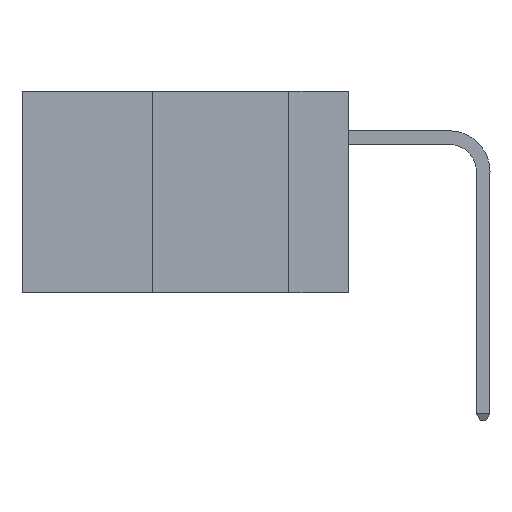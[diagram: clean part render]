
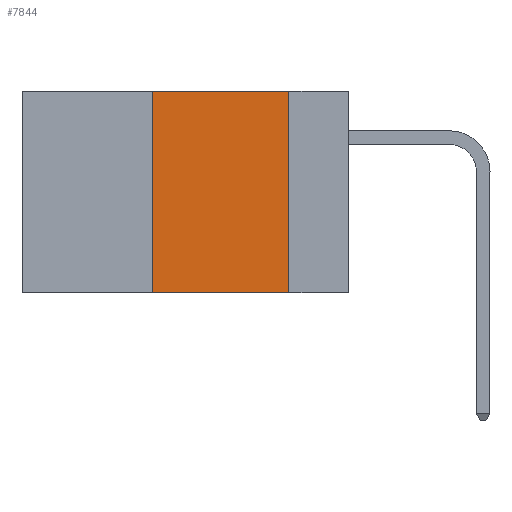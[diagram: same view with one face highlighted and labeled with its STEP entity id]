
A CAD part, left-side view. The second image highlights one B-rep face of the part: STEP entity #7844.
In plain terms, the highlighted planar face has unit normal (-1, 0, 0).
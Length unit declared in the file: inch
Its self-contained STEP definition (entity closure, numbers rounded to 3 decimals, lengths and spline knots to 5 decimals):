
#336 = ORIENTED_EDGE ( 'NONE', *, *, #8091, .F. ) ;
#542 = LINE ( 'NONE', #5644, #5907 ) ;
#557 = EDGE_CURVE ( 'NONE', #7645, #10335, #3530, .T. ) ;
#915 = VERTEX_POINT ( 'NONE', #5698 ) ;
#1293 = DIRECTION ( 'NONE',  ( 0., 0., 1. ) ) ;
#1520 = DIRECTION ( 'NONE',  ( 0., 0., -1. ) ) ;
#2059 = FACE_OUTER_BOUND ( 'NONE', #9826, .T. ) ;
#2128 = VERTEX_POINT ( 'NONE', #10672 ) ;
#2358 = CARTESIAN_POINT ( 'NONE',  ( 0., 0.36, 0. ) ) ;
#2717 = DIRECTION ( 'NONE',  ( 0., 0., -1. ) ) ;
#3252 = EDGE_CURVE ( 'NONE', #2128, #915, #4286, .T. ) ;
#3378 = DIRECTION ( 'NONE',  ( 0., -1., 0. ) ) ;
#3530 = LINE ( 'NONE', #12427, #5040 ) ;
#3642 = ORIENTED_EDGE ( 'NONE', *, *, #7316, .T. ) ;
#4110 = VECTOR ( 'NONE', #3378, 39.37008 ) ;
#4262 = LINE ( 'NONE', #7704, #4110 ) ;
#4286 = LINE ( 'NONE', #2358, #6313 ) ;
#4820 = DIRECTION ( 'NONE',  ( 1., 0., 0. ) ) ;
#5040 = VECTOR ( 'NONE', #2717, 39.37008 ) ;
#5265 = AXIS2_PLACEMENT_3D ( 'NONE', #8032, #4820, #1520 ) ;
#5311 = ORIENTED_EDGE ( 'NONE', *, *, #557, .F. ) ;
#5644 = CARTESIAN_POINT ( 'NONE',  ( 0., 0.6, 0. ) ) ;
#5698 = CARTESIAN_POINT ( 'NONE',  ( 0., 0.36, 0. ) ) ;
#5907 = VECTOR ( 'NONE', #9895, 39.37008 ) ;
#6313 = VECTOR ( 'NONE', #1293, 39.37008 ) ;
#6611 = CARTESIAN_POINT ( 'NONE',  ( 0., 0.11, 0. ) ) ;
#7316 = EDGE_CURVE ( 'NONE', #2128, #10335, #4262, .T. ) ;
#7645 = VERTEX_POINT ( 'NONE', #6611 ) ;
#7704 = CARTESIAN_POINT ( 'NONE',  ( 0., 0.6, -0.37 ) ) ;
#7844 = ADVANCED_FACE ( 'NONE', ( #2059 ), #7970, .F. ) ;
#7970 = PLANE ( 'NONE',  #5265 ) ;
#8032 = CARTESIAN_POINT ( 'NONE',  ( 0., 0.6, 0. ) ) ;
#8091 = EDGE_CURVE ( 'NONE', #915, #7645, #542, .T. ) ;
#9826 = EDGE_LOOP ( 'NONE', ( #5311, #336, #9958, #3642 ) ) ;
#9895 = DIRECTION ( 'NONE',  ( 0., -1., 0. ) ) ;
#9958 = ORIENTED_EDGE ( 'NONE', *, *, #3252, .F. ) ;
#10335 = VERTEX_POINT ( 'NONE', #12921 ) ;
#10672 = CARTESIAN_POINT ( 'NONE',  ( 0., 0.36, -0.37 ) ) ;
#12427 = CARTESIAN_POINT ( 'NONE',  ( 0., 0.11, 0. ) ) ;
#12921 = CARTESIAN_POINT ( 'NONE',  ( 0., 0.11, -0.37 ) ) ;
